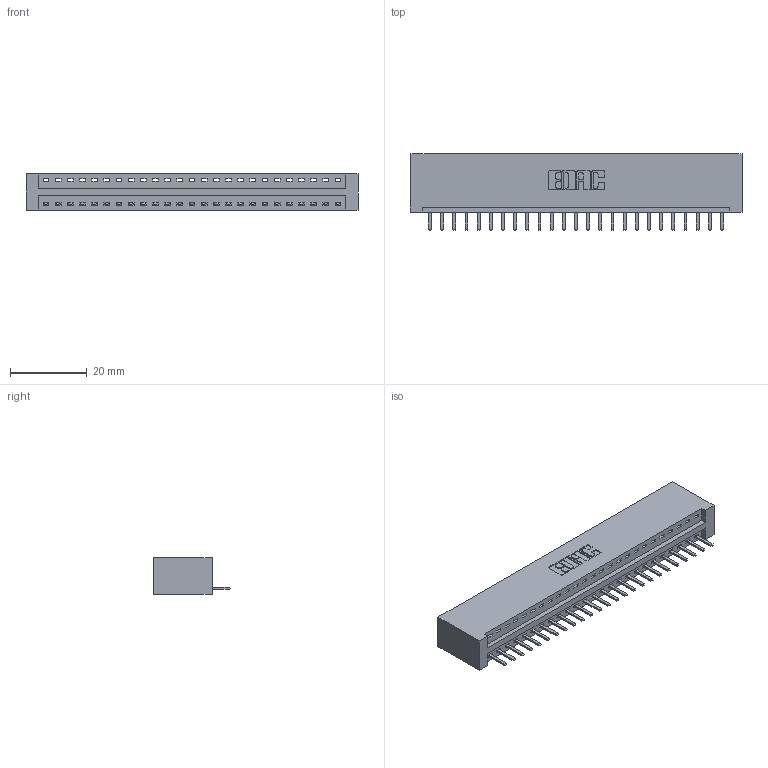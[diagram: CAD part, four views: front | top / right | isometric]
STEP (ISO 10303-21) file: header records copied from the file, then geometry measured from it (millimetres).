
FILE_DESCRIPTION (( 'STEP AP203' ), '1' );
FILE_NAME ('396-025-520-101.STEP', '2018-09-01T15:49:09', ( '' ), ( '' ), 'SwSTEP 2.0', 'SolidWorks 2016', '' );
FILE_SCHEMA (( 'CONFIG_CONTROL_DESIGN' ));
Length unit declared in the file: inch
Products named in the file (3): 345-292-001_345-293-120; 396-025-520-101; 346 Part_No Mounting Lugs
Assembly tree (26 placements, depth 2):
  396-025-520-101
    346 Part_No Mounting Lugs
    345-292-001_345-293-120  x25
Bounding box: 86.61 x 20.02 x 9.4 mm (x, y, z)
Volume: 8651.2 mm3; surface area: 10464.5 mm2
Topology: 26 solids, 26 shells, 1664 faces, 4905 edges, 3202 vertices
Faces by surface type: plane 1122, cylinder 542
Entity records: 17641 total; most frequent: CARTESIAN_POINT 3047, ORIENTED_EDGE 2994, DIRECTION 2691, EDGE_CURVE 1497, VECTOR 1269, LINE 1269, VERTEX_POINT 994, AXIS2_PLACEMENT_3D 711
